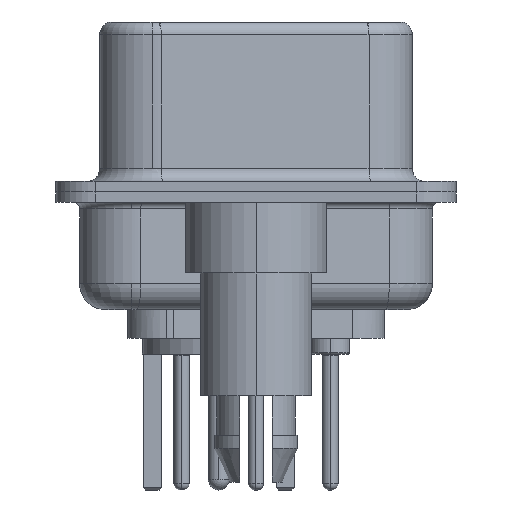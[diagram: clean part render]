
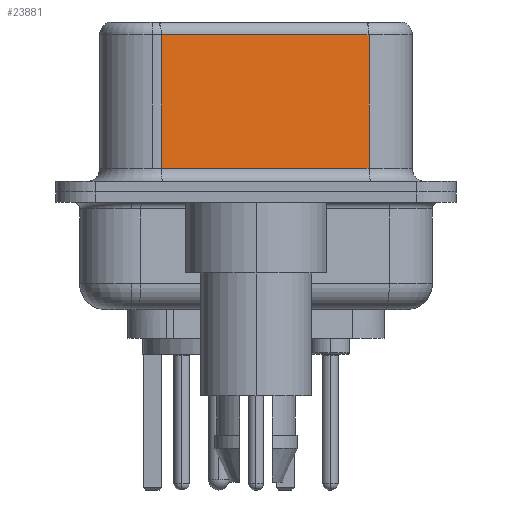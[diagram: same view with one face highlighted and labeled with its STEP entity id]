
A CAD part, left-side view. The second image highlights one B-rep face of the part: STEP entity #23881.
In plain terms, the highlighted planar face has unit normal (-0.985, -0.174, 0).
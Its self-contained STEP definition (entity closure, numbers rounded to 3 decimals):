
#5 = ORIENTED_EDGE ( 'NONE', *, *, #8170, .F. ) ;
#633 = VERTEX_POINT ( 'NONE', #26181 ) ;
#958 = VERTEX_POINT ( 'NONE', #2837 ) ;
#1359 = VECTOR ( 'NONE', #24233, 1000. ) ;
#1475 = CARTESIAN_POINT ( 'NONE',  ( 5.132, -4.322, 6.52 ) ) ;
#1742 = CARTESIAN_POINT ( 'NONE',  ( 5.132, -4.322, 6.02 ) ) ;
#2837 = CARTESIAN_POINT ( 'NONE',  ( 5.132, -4.322, 6.02 ) ) ;
#4743 = VERTEX_POINT ( 'NONE', #19442 ) ;
#5000 = EDGE_CURVE ( 'NONE', #958, #20899, #29584, .T. ) ;
#5494 = ORIENTED_EDGE ( 'NONE', *, *, #5000, .T. ) ;
#5783 = DIRECTION ( 'NONE',  ( 0.174, -0.985, 0. ) ) ;
#5956 = AXIS2_PLACEMENT_3D ( 'NONE', #1475, #19818, #6075 ) ;
#6075 = DIRECTION ( 'NONE',  ( -0.174, 0.985, 0. ) ) ;
#6996 = EDGE_LOOP ( 'NONE', ( #5, #5494, #27340, #24701 ) ) ;
#8170 = EDGE_CURVE ( 'NONE', #958, #4743, #14220, .T. ) ;
#10328 = CARTESIAN_POINT ( 'NONE',  ( 5.132, -4.322, 0.9 ) ) ;
#10418 = CARTESIAN_POINT ( 'NONE',  ( 5.132, -4.322, 6.52 ) ) ;
#12862 = PLANE ( 'NONE',  #5956 ) ;
#13625 = VECTOR ( 'NONE', #28347, 1000. ) ;
#14220 = LINE ( 'NONE', #10418, #1359 ) ;
#16443 = FACE_OUTER_BOUND ( 'NONE', #6996, .T. ) ;
#16783 = VECTOR ( 'NONE', #5783, 1000. ) ;
#16813 = CARTESIAN_POINT ( 'NONE',  ( 3.73, 3.628, 6.52 ) ) ;
#17336 = EDGE_CURVE ( 'NONE', #633, #4743, #29077, .T. ) ;
#19442 = CARTESIAN_POINT ( 'NONE',  ( 5.132, -4.322, 0.9 ) ) ;
#19818 = DIRECTION ( 'NONE',  ( 0.985, 0.174, 0. ) ) ;
#20899 = VERTEX_POINT ( 'NONE', #27450 ) ;
#21269 = LINE ( 'NONE', #16813, #13625 ) ;
#22825 = VECTOR ( 'NONE', #24116, 1000. ) ;
#23881 = ADVANCED_FACE ( 'NONE', ( #16443 ), #12862, .F. ) ;
#24116 = DIRECTION ( 'NONE',  ( -0.174, 0.985, 0. ) ) ;
#24233 = DIRECTION ( 'NONE',  ( 0., 0., -1. ) ) ;
#24701 = ORIENTED_EDGE ( 'NONE', *, *, #17336, .T. ) ;
#26181 = CARTESIAN_POINT ( 'NONE',  ( 3.73, 3.628, 0.9 ) ) ;
#27340 = ORIENTED_EDGE ( 'NONE', *, *, #29606, .T. ) ;
#27450 = CARTESIAN_POINT ( 'NONE',  ( 3.73, 3.628, 6.02 ) ) ;
#28347 = DIRECTION ( 'NONE',  ( 0., 0., -1. ) ) ;
#29077 = LINE ( 'NONE', #10328, #16783 ) ;
#29584 = LINE ( 'NONE', #1742, #22825 ) ;
#29606 = EDGE_CURVE ( 'NONE', #20899, #633, #21269, .T. ) ;
